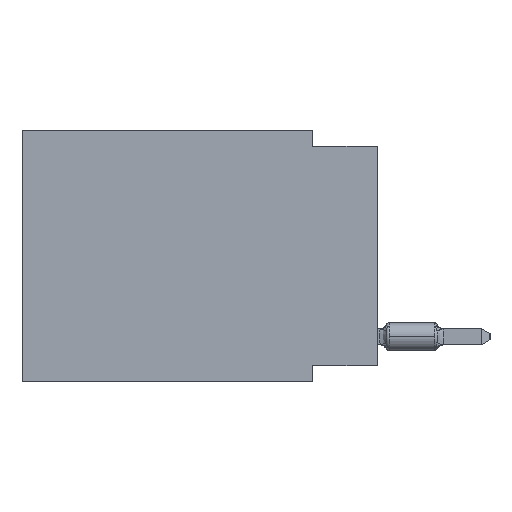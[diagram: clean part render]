
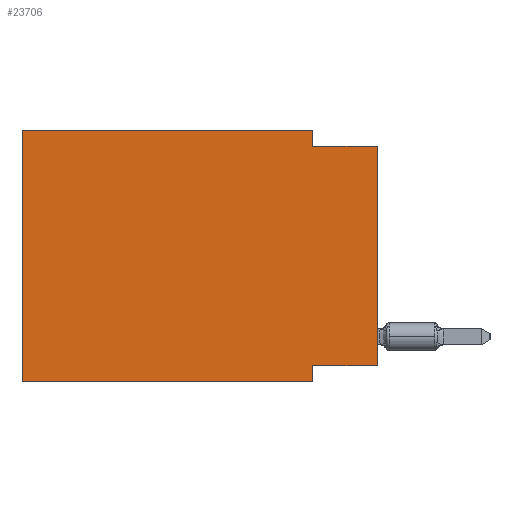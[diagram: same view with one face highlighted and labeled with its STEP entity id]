
A CAD part, left-side view. The second image highlights one B-rep face of the part: STEP entity #23706.
In plain terms, the highlighted planar face has unit normal (-1, 0, 0).
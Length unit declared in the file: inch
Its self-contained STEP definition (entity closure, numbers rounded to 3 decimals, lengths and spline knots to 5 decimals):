
#437 = CARTESIAN_POINT ( 'NONE',  ( 0., 0.55, 0. ) ) ;
#873 = VERTEX_POINT ( 'NONE', #30030 ) ;
#1558 = CARTESIAN_POINT ( 'NONE',  ( 0., 0.55, -0.39 ) ) ;
#2652 = CARTESIAN_POINT ( 'NONE',  ( 0., 0.1, -0.365 ) ) ;
#3130 = DIRECTION ( 'NONE',  ( 0., 0., -1. ) ) ;
#3204 = VERTEX_POINT ( 'NONE', #2652 ) ;
#3235 = CARTESIAN_POINT ( 'NONE',  ( 0., 0.1, 0. ) ) ;
#5266 = CARTESIAN_POINT ( 'NONE',  ( 0., 0.55, -0.39 ) ) ;
#5343 = CARTESIAN_POINT ( 'NONE',  ( 0., 0.1, 0. ) ) ;
#5947 = LINE ( 'NONE', #5343, #32435 ) ;
#6728 = LINE ( 'NONE', #437, #20702 ) ;
#6735 = DIRECTION ( 'NONE',  ( 1., 0., 0. ) ) ;
#7390 = VECTOR ( 'NONE', #13760, 39.37008 ) ;
#9229 = CARTESIAN_POINT ( 'NONE',  ( 0., 0.1, -0.39 ) ) ;
#9554 = VERTEX_POINT ( 'NONE', #1558 ) ;
#9789 = PLANE ( 'NONE',  #26571 ) ;
#9925 = LINE ( 'NONE', #25745, #7390 ) ;
#11450 = VERTEX_POINT ( 'NONE', #36441 ) ;
#11982 = CARTESIAN_POINT ( 'NONE',  ( 0., 0., -0.025 ) ) ;
#13760 = DIRECTION ( 'NONE',  ( 0., 0., 1. ) ) ;
#13832 = VERTEX_POINT ( 'NONE', #24256 ) ;
#14041 = EDGE_CURVE ( 'NONE', #3204, #873, #37071, .T. ) ;
#14968 = ORIENTED_EDGE ( 'NONE', *, *, #25154, .T. ) ;
#16462 = CARTESIAN_POINT ( 'NONE',  ( 0., 0., -0.365 ) ) ;
#18162 = EDGE_LOOP ( 'NONE', ( #19890, #29579, #18224, #24795, #24989, #14968, #25221, #30402 ) ) ;
#18224 = ORIENTED_EDGE ( 'NONE', *, *, #23529, .F. ) ;
#18792 = VECTOR ( 'NONE', #23946, 39.37008 ) ;
#19890 = ORIENTED_EDGE ( 'NONE', *, *, #26511, .T. ) ;
#20702 = VECTOR ( 'NONE', #28465, 39.37008 ) ;
#20897 = CARTESIAN_POINT ( 'NONE',  ( 0., 0., 0. ) ) ;
#21367 = DIRECTION ( 'NONE',  ( 0., 0., -1. ) ) ;
#21971 = LINE ( 'NONE', #28466, #27846 ) ;
#22503 = EDGE_CURVE ( 'NONE', #22600, #3204, #21971, .T. ) ;
#22600 = VERTEX_POINT ( 'NONE', #16462 ) ;
#22730 = VECTOR ( 'NONE', #35933, 39.37008 ) ;
#22959 = DIRECTION ( 'NONE',  ( 0., 1., 0. ) ) ;
#23529 = EDGE_CURVE ( 'NONE', #37554, #11450, #5947, .T. ) ;
#23706 = ADVANCED_FACE ( 'NONE', ( #34957 ), #9789, .F. ) ;
#23946 = DIRECTION ( 'NONE',  ( 0., -1., 0. ) ) ;
#24256 = CARTESIAN_POINT ( 'NONE',  ( 0., 0.55, 0. ) ) ;
#24543 = VECTOR ( 'NONE', #3130, 39.37008 ) ;
#24795 = ORIENTED_EDGE ( 'NONE', *, *, #38346, .F. ) ;
#24989 = ORIENTED_EDGE ( 'NONE', *, *, #30023, .F. ) ;
#25154 = EDGE_CURVE ( 'NONE', #9554, #873, #36335, .T. ) ;
#25221 = ORIENTED_EDGE ( 'NONE', *, *, #14041, .F. ) ;
#25745 = CARTESIAN_POINT ( 'NONE',  ( 0., 0.55, 0. ) ) ;
#26511 = EDGE_CURVE ( 'NONE', #22600, #32392, #33095, .T. ) ;
#26571 = AXIS2_PLACEMENT_3D ( 'NONE', #34571, #6735, #31520 ) ;
#27846 = VECTOR ( 'NONE', #22959, 39.37008 ) ;
#28465 = DIRECTION ( 'NONE',  ( 0., -1., 0. ) ) ;
#28466 = CARTESIAN_POINT ( 'NONE',  ( 0., 0., -0.365 ) ) ;
#29579 = ORIENTED_EDGE ( 'NONE', *, *, #39718, .F. ) ;
#29906 = VECTOR ( 'NONE', #33291, 39.37008 ) ;
#30023 = EDGE_CURVE ( 'NONE', #9554, #13832, #9925, .T. ) ;
#30030 = CARTESIAN_POINT ( 'NONE',  ( 0., 0.1, -0.39 ) ) ;
#30402 = ORIENTED_EDGE ( 'NONE', *, *, #22503, .F. ) ;
#31520 = DIRECTION ( 'NONE',  ( 0., 0., -1. ) ) ;
#32392 = VERTEX_POINT ( 'NONE', #11982 ) ;
#32435 = VECTOR ( 'NONE', #21367, 39.37008 ) ;
#33095 = LINE ( 'NONE', #20897, #29906 ) ;
#33291 = DIRECTION ( 'NONE',  ( 0., 0., 1. ) ) ;
#34571 = CARTESIAN_POINT ( 'NONE',  ( 0., 0.55, 0. ) ) ;
#34957 = FACE_OUTER_BOUND ( 'NONE', #18162, .T. ) ;
#35933 = DIRECTION ( 'NONE',  ( 0., -1., 0. ) ) ;
#36335 = LINE ( 'NONE', #5266, #18792 ) ;
#36441 = CARTESIAN_POINT ( 'NONE',  ( 0., 0.1, -0.025 ) ) ;
#37071 = LINE ( 'NONE', #9229, #24543 ) ;
#37554 = VERTEX_POINT ( 'NONE', #3235 ) ;
#38346 = EDGE_CURVE ( 'NONE', #13832, #37554, #6728, .T. ) ;
#39408 = CARTESIAN_POINT ( 'NONE',  ( 0., 0., -0.025 ) ) ;
#39718 = EDGE_CURVE ( 'NONE', #11450, #32392, #39810, .T. ) ;
#39810 = LINE ( 'NONE', #39408, #22730 ) ;
